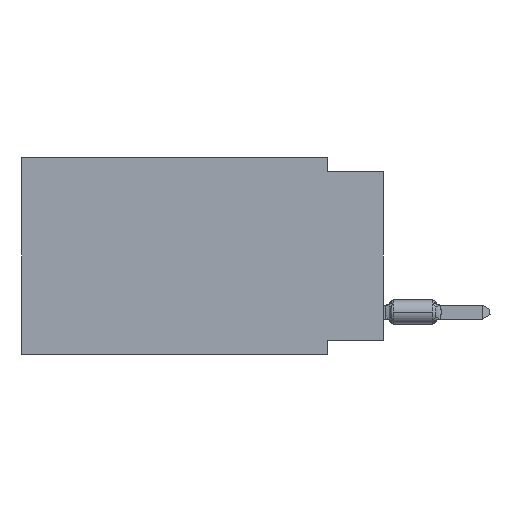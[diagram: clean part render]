
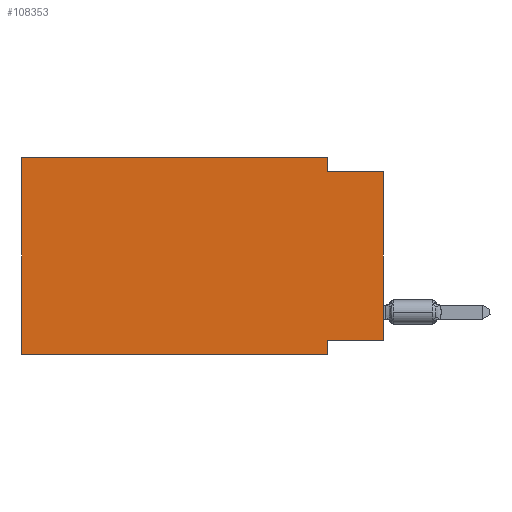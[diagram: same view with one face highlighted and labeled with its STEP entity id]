
A CAD part, left-side view. The second image highlights one B-rep face of the part: STEP entity #108353.
In plain terms, the highlighted planar face has unit normal (-1, 0, 0).
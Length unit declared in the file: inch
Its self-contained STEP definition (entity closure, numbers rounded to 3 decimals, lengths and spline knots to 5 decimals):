
#3194 = CARTESIAN_POINT ( 'NONE',  ( 0., 0.645, -0.35 ) ) ;
#5522 = VERTEX_POINT ( 'NONE', #80952 ) ;
#8346 = VECTOR ( 'NONE', #49160, 39.37008 ) ;
#9412 = EDGE_CURVE ( 'NONE', #13385, #102670, #14384, .T. ) ;
#10182 = VERTEX_POINT ( 'NONE', #102750 ) ;
#10977 = CARTESIAN_POINT ( 'NONE',  ( 0., 0.1, -0.35 ) ) ;
#13385 = VERTEX_POINT ( 'NONE', #97125 ) ;
#13405 = DIRECTION ( 'NONE',  ( 0., -1., 0. ) ) ;
#13755 = VECTOR ( 'NONE', #70238, 39.37008 ) ;
#14002 = LINE ( 'NONE', #103958, #65284 ) ;
#14384 = LINE ( 'NONE', #106099, #13755 ) ;
#15998 = CARTESIAN_POINT ( 'NONE',  ( 0., 0.1, -0.325 ) ) ;
#21965 = DIRECTION ( 'NONE',  ( 0., -1., 0. ) ) ;
#23385 = DIRECTION ( 'NONE',  ( 0., 0., -1. ) ) ;
#26148 = ORIENTED_EDGE ( 'NONE', *, *, #49633, .F. ) ;
#28804 = AXIS2_PLACEMENT_3D ( 'NONE', #68660, #115068, #47662 ) ;
#29655 = LINE ( 'NONE', #63798, #82117 ) ;
#32530 = VECTOR ( 'NONE', #21965, 39.37008 ) ;
#33833 = DIRECTION ( 'NONE',  ( 0., 1., 0. ) ) ;
#34747 = DIRECTION ( 'NONE',  ( 0., 0., 1. ) ) ;
#36062 = VECTOR ( 'NONE', #33833, 39.37008 ) ;
#37698 = CARTESIAN_POINT ( 'NONE',  ( 0., 0.1, 0. ) ) ;
#37714 = VECTOR ( 'NONE', #13405, 39.37008 ) ;
#38140 = VECTOR ( 'NONE', #34747, 39.37008 ) ;
#40267 = EDGE_CURVE ( 'NONE', #10182, #57306, #83780, .T. ) ;
#41048 = CARTESIAN_POINT ( 'NONE',  ( 0., 0.645, 0. ) ) ;
#42103 = LINE ( 'NONE', #60310, #36062 ) ;
#43294 = EDGE_CURVE ( 'NONE', #101910, #57306, #56266, .T. ) ;
#43480 = ORIENTED_EDGE ( 'NONE', *, *, #65612, .F. ) ;
#46166 = DIRECTION ( 'NONE',  ( 0., 0., 1. ) ) ;
#47662 = DIRECTION ( 'NONE',  ( 0., 0., -1. ) ) ;
#49160 = DIRECTION ( 'NONE',  ( 0., 0., -1. ) ) ;
#49633 = EDGE_CURVE ( 'NONE', #98672, #101910, #42103, .T. ) ;
#51044 = LINE ( 'NONE', #41048, #37714 ) ;
#56266 = LINE ( 'NONE', #10977, #8346 ) ;
#56880 = ORIENTED_EDGE ( 'NONE', *, *, #43294, .F. ) ;
#57306 = VERTEX_POINT ( 'NONE', #107472 ) ;
#60310 = CARTESIAN_POINT ( 'NONE',  ( 0., 0., -0.325 ) ) ;
#63798 = CARTESIAN_POINT ( 'NONE',  ( 0., 0.645, 0. ) ) ;
#65284 = VECTOR ( 'NONE', #23385, 39.37008 ) ;
#65612 = EDGE_CURVE ( 'NONE', #10182, #5522, #29655, .T. ) ;
#68660 = CARTESIAN_POINT ( 'NONE',  ( 0., 0.645, 0. ) ) ;
#69211 = PLANE ( 'NONE',  #28804 ) ;
#69282 = ORIENTED_EDGE ( 'NONE', *, *, #70624, .F. ) ;
#70032 = CARTESIAN_POINT ( 'NONE',  ( 0., 0., 0. ) ) ;
#70238 = DIRECTION ( 'NONE',  ( 0., -1., 0. ) ) ;
#70624 = EDGE_CURVE ( 'NONE', #5522, #102048, #51044, .T. ) ;
#72632 = ORIENTED_EDGE ( 'NONE', *, *, #82074, .T. ) ;
#76081 = ORIENTED_EDGE ( 'NONE', *, *, #90697, .F. ) ;
#76478 = CARTESIAN_POINT ( 'NONE',  ( 0., 0., -0.025 ) ) ;
#80952 = CARTESIAN_POINT ( 'NONE',  ( 0., 0.645, 0. ) ) ;
#81184 = LINE ( 'NONE', #70032, #38140 ) ;
#82074 = EDGE_CURVE ( 'NONE', #98672, #102670, #81184, .T. ) ;
#82117 = VECTOR ( 'NONE', #46166, 39.37008 ) ;
#83780 = LINE ( 'NONE', #3194, #32530 ) ;
#90697 = EDGE_CURVE ( 'NONE', #102048, #13385, #14002, .T. ) ;
#90942 = CARTESIAN_POINT ( 'NONE',  ( 0., 0., -0.325 ) ) ;
#97125 = CARTESIAN_POINT ( 'NONE',  ( 0., 0.1, -0.025 ) ) ;
#98672 = VERTEX_POINT ( 'NONE', #90942 ) ;
#100066 = ORIENTED_EDGE ( 'NONE', *, *, #40267, .T. ) ;
#101910 = VERTEX_POINT ( 'NONE', #15998 ) ;
#102048 = VERTEX_POINT ( 'NONE', #37698 ) ;
#102670 = VERTEX_POINT ( 'NONE', #76478 ) ;
#102750 = CARTESIAN_POINT ( 'NONE',  ( 0., 0.645, -0.35 ) ) ;
#103958 = CARTESIAN_POINT ( 'NONE',  ( 0., 0.1, 0. ) ) ;
#106099 = CARTESIAN_POINT ( 'NONE',  ( 0., 0., -0.025 ) ) ;
#106239 = FACE_OUTER_BOUND ( 'NONE', #111112, .T. ) ;
#107472 = CARTESIAN_POINT ( 'NONE',  ( 0., 0.1, -0.35 ) ) ;
#108353 = ADVANCED_FACE ( 'NONE', ( #106239 ), #69211, .F. ) ;
#111112 = EDGE_LOOP ( 'NONE', ( #72632, #114828, #76081, #69282, #43480, #100066, #56880, #26148 ) ) ;
#114828 = ORIENTED_EDGE ( 'NONE', *, *, #9412, .F. ) ;
#115068 = DIRECTION ( 'NONE',  ( 1., 0., 0. ) ) ;
